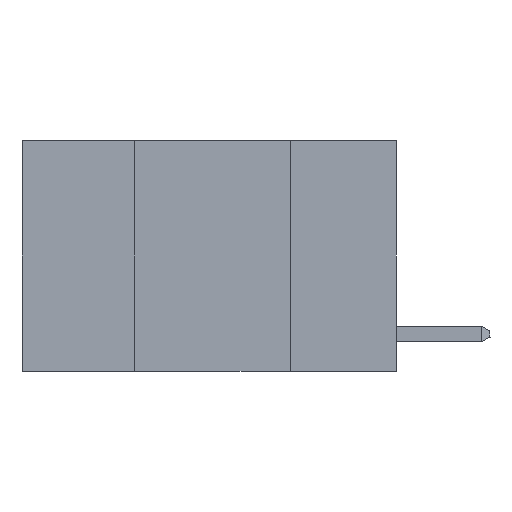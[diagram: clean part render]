
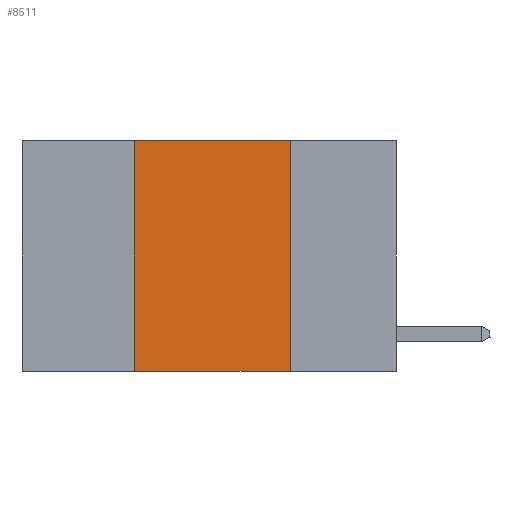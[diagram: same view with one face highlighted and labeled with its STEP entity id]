
A CAD part, left-side view. The second image highlights one B-rep face of the part: STEP entity #8511.
In plain terms, the highlighted planar face has unit normal (-1, 0, 0).
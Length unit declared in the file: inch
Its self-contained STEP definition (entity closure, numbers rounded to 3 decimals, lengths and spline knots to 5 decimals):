
#271 = CARTESIAN_POINT ( 'NONE',  ( 0., 0.6, 0. ) ) ;
#1966 = DIRECTION ( 'NONE',  ( 0., -1., 0. ) ) ;
#2462 = EDGE_CURVE ( 'NONE', #9253, #12080, #2863, .T. ) ;
#2863 = LINE ( 'NONE', #25232, #8485 ) ;
#3454 = VERTEX_POINT ( 'NONE', #5028 ) ;
#4439 = AXIS2_PLACEMENT_3D ( 'NONE', #271, #27778, #14053 ) ;
#4856 = EDGE_LOOP ( 'NONE', ( #20634, #14909, #6503, #23767 ) ) ;
#5028 = CARTESIAN_POINT ( 'NONE',  ( 0., 0.17, -0.37 ) ) ;
#5789 = LINE ( 'NONE', #15334, #23291 ) ;
#6503 = ORIENTED_EDGE ( 'NONE', *, *, #2462, .F. ) ;
#6632 = FACE_OUTER_BOUND ( 'NONE', #4856, .T. ) ;
#8426 = DIRECTION ( 'NONE',  ( 0., 0., -1. ) ) ;
#8485 = VECTOR ( 'NONE', #9430, 39.37008 ) ;
#8511 = ADVANCED_FACE ( 'NONE', ( #6632 ), #27681, .F. ) ;
#8769 = CARTESIAN_POINT ( 'NONE',  ( 0., 0.42, -0.37 ) ) ;
#9253 = VERTEX_POINT ( 'NONE', #8769 ) ;
#9430 = DIRECTION ( 'NONE',  ( 0., 0., 1. ) ) ;
#9967 = LINE ( 'NONE', #10743, #23830 ) ;
#10743 = CARTESIAN_POINT ( 'NONE',  ( 0., 0.6, -0.37 ) ) ;
#12080 = VERTEX_POINT ( 'NONE', #16893 ) ;
#14053 = DIRECTION ( 'NONE',  ( 0., 0., -1. ) ) ;
#14909 = ORIENTED_EDGE ( 'NONE', *, *, #24752, .F. ) ;
#15334 = CARTESIAN_POINT ( 'NONE',  ( 0., 0.17, 0. ) ) ;
#16371 = LINE ( 'NONE', #20164, #28114 ) ;
#16893 = CARTESIAN_POINT ( 'NONE',  ( 0., 0.42, 0. ) ) ;
#20141 = CARTESIAN_POINT ( 'NONE',  ( 0., 0.17, 0. ) ) ;
#20164 = CARTESIAN_POINT ( 'NONE',  ( 0., 0.6, 0. ) ) ;
#20634 = ORIENTED_EDGE ( 'NONE', *, *, #27456, .F. ) ;
#23291 = VECTOR ( 'NONE', #8426, 39.37008 ) ;
#23767 = ORIENTED_EDGE ( 'NONE', *, *, #24493, .T. ) ;
#23830 = VECTOR ( 'NONE', #26666, 39.37008 ) ;
#24493 = EDGE_CURVE ( 'NONE', #9253, #3454, #9967, .T. ) ;
#24752 = EDGE_CURVE ( 'NONE', #12080, #28231, #16371, .T. ) ;
#25232 = CARTESIAN_POINT ( 'NONE',  ( 0., 0.42, 0. ) ) ;
#26666 = DIRECTION ( 'NONE',  ( 0., -1., 0. ) ) ;
#27456 = EDGE_CURVE ( 'NONE', #28231, #3454, #5789, .T. ) ;
#27681 = PLANE ( 'NONE',  #4439 ) ;
#27778 = DIRECTION ( 'NONE',  ( 1., 0., 0. ) ) ;
#28114 = VECTOR ( 'NONE', #1966, 39.37008 ) ;
#28231 = VERTEX_POINT ( 'NONE', #20141 ) ;
